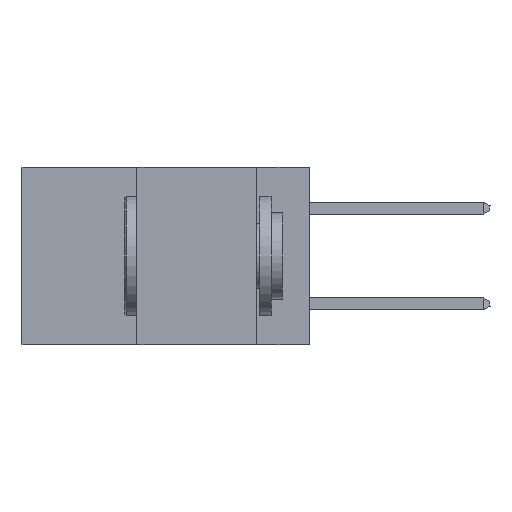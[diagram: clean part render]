
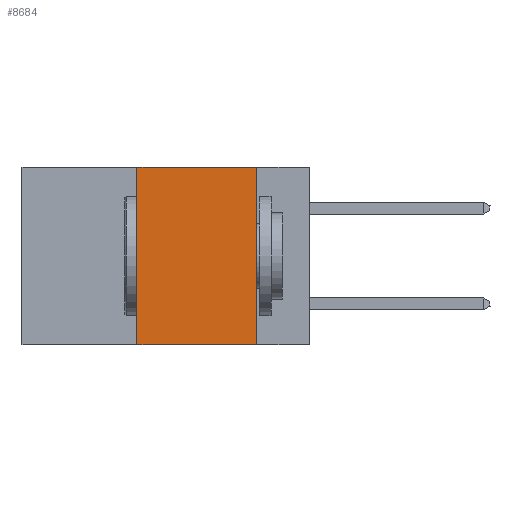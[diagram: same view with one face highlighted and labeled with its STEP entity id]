
A CAD part, left-side view. The second image highlights one B-rep face of the part: STEP entity #8684.
In plain terms, the highlighted planar face has unit normal (-1, 0, 0).
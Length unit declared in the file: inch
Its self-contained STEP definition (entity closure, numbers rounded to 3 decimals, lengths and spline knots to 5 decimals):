
#104 = CARTESIAN_POINT ( 'NONE',  ( 0., 0.36, 0. ) ) ;
#1706 = DIRECTION ( 'NONE',  ( 0., 0., -1. ) ) ;
#3993 = EDGE_CURVE ( 'NONE', #25610, #18342, #5631, .T. ) ;
#4861 = EDGE_LOOP ( 'NONE', ( #13167, #22214, #29969, #13622 ) ) ;
#4873 = VECTOR ( 'NONE', #23096, 39.37008 ) ;
#5045 = VECTOR ( 'NONE', #19030, 39.37008 ) ;
#5373 = CARTESIAN_POINT ( 'NONE',  ( 0., 0.11, 0. ) ) ;
#5631 = LINE ( 'NONE', #11420, #4873 ) ;
#6700 = VERTEX_POINT ( 'NONE', #13940 ) ;
#6856 = EDGE_CURVE ( 'NONE', #25610, #28416, #30004, .T. ) ;
#8684 = ADVANCED_FACE ( 'NONE', ( #10532 ), #11220, .F. ) ;
#9326 = EDGE_CURVE ( 'NONE', #18342, #6700, #23957, .T. ) ;
#10187 = DIRECTION ( 'NONE',  ( 0., 0., -1. ) ) ;
#10532 = FACE_OUTER_BOUND ( 'NONE', #4861, .T. ) ;
#11220 = PLANE ( 'NONE',  #24178 ) ;
#11420 = CARTESIAN_POINT ( 'NONE',  ( 0., 0.36, 0. ) ) ;
#12097 = CARTESIAN_POINT ( 'NONE',  ( 0., 0.6, -0.37 ) ) ;
#12932 = LINE ( 'NONE', #5373, #13662 ) ;
#13167 = ORIENTED_EDGE ( 'NONE', *, *, #27619, .F. ) ;
#13622 = ORIENTED_EDGE ( 'NONE', *, *, #6856, .T. ) ;
#13662 = VECTOR ( 'NONE', #10187, 39.37008 ) ;
#13940 = CARTESIAN_POINT ( 'NONE',  ( 0., 0.11, 0. ) ) ;
#15906 = DIRECTION ( 'NONE',  ( 1., 0., 0. ) ) ;
#18131 = DIRECTION ( 'NONE',  ( 0., -1., 0. ) ) ;
#18342 = VERTEX_POINT ( 'NONE', #104 ) ;
#19030 = DIRECTION ( 'NONE',  ( 0., -1., 0. ) ) ;
#19597 = CARTESIAN_POINT ( 'NONE',  ( 0., 0.36, -0.37 ) ) ;
#22214 = ORIENTED_EDGE ( 'NONE', *, *, #9326, .F. ) ;
#23096 = DIRECTION ( 'NONE',  ( 0., 0., 1. ) ) ;
#23957 = LINE ( 'NONE', #29749, #29469 ) ;
#24178 = AXIS2_PLACEMENT_3D ( 'NONE', #29891, #15906, #1706 ) ;
#25610 = VERTEX_POINT ( 'NONE', #19597 ) ;
#26826 = CARTESIAN_POINT ( 'NONE',  ( 0., 0.11, -0.37 ) ) ;
#27619 = EDGE_CURVE ( 'NONE', #6700, #28416, #12932, .T. ) ;
#28416 = VERTEX_POINT ( 'NONE', #26826 ) ;
#29469 = VECTOR ( 'NONE', #18131, 39.37008 ) ;
#29749 = CARTESIAN_POINT ( 'NONE',  ( 0., 0.6, 0. ) ) ;
#29891 = CARTESIAN_POINT ( 'NONE',  ( 0., 0.6, 0. ) ) ;
#29969 = ORIENTED_EDGE ( 'NONE', *, *, #3993, .F. ) ;
#30004 = LINE ( 'NONE', #12097, #5045 ) ;
